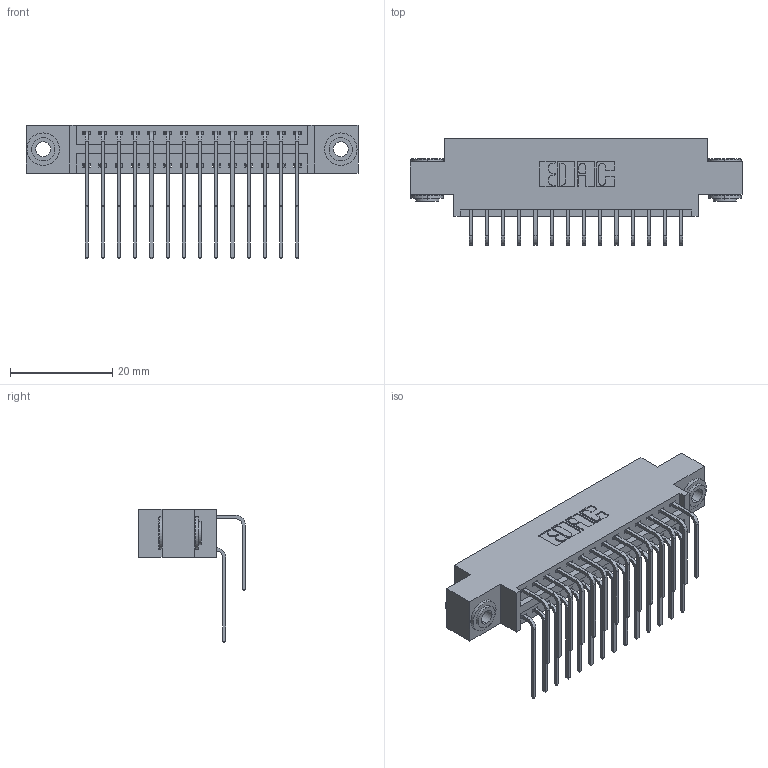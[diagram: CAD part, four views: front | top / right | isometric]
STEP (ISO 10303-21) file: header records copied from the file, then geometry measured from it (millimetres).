
FILE_DESCRIPTION (( 'STEP AP203' ), '1' );
FILE_NAME ('396-028-559-803.STEP', '2019-11-03T06:24:56', ( '' ), ( '' ), 'SwSTEP 2.0', 'SolidWorks 2016', '' );
FILE_SCHEMA (( 'CONFIG_CONTROL_DESIGN' ));
Length unit declared in the file: inch
Products named in the file (5): 345-292-001_559 Tail - 2; 345-250-002_345-250-002-102; 345-292-001_558 559 Tail - 1; 396-028-559-803; 346 Part_0.170 Offset - 0.156 Dia-TH
Assembly tree (31 placements, depth 2):
  396-028-559-803
    346 Part_0.170 Offset - 0.156 Dia-TH
    345-292-001_558 559 Tail - 1  x14
    345-292-001_559 Tail - 2  x14
    345-250-002_345-250-002-102  x2
Bounding box: 65.02 x 20.89 x 26.16 mm (x, y, z)
Volume: 6149.5 mm3; surface area: 9181.5 mm2
Topology: 31 solids, 31 shells, 1676 faces, 4925 edges, 3242 vertices
Faces by surface type: plane 1126, cylinder 542, cone 8
Entity records: 15472 total; most frequent: CARTESIAN_POINT 2618, ORIENTED_EDGE 2494, DIRECTION 2361, EDGE_CURVE 1247, LINE 995, VECTOR 995, VERTEX_POINT 826, AXIS2_PLACEMENT_3D 683
